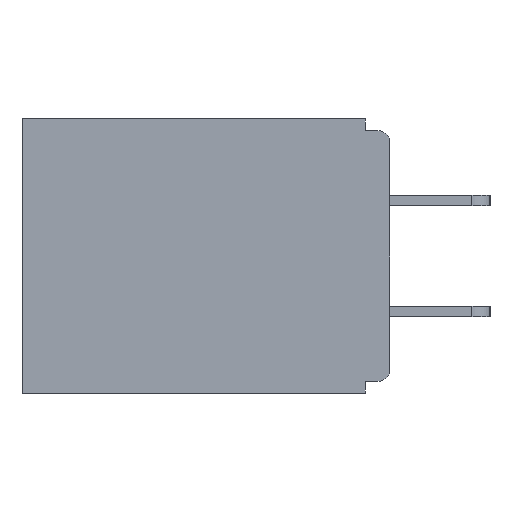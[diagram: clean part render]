
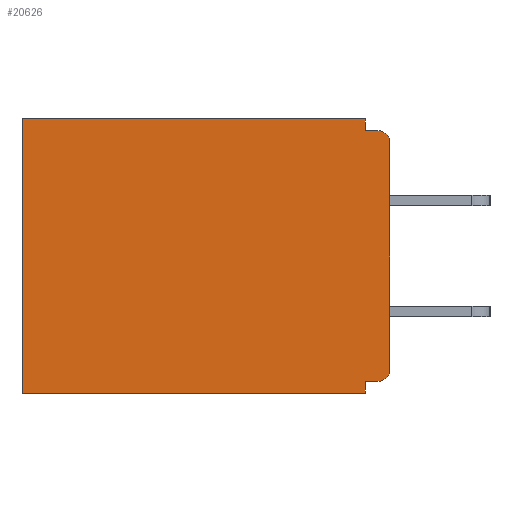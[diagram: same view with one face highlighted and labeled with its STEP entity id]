
A CAD part, left-side view. The second image highlights one B-rep face of the part: STEP entity #20626.
In plain terms, the highlighted planar face has unit normal (-1, 0, 0).
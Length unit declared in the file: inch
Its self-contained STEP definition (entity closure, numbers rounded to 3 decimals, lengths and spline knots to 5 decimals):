
#34 = DIRECTION ( 'NONE',  ( 0., -1., 0. ) ) ;
#69 = VERTEX_POINT ( 'NONE', #23006 ) ;
#91 = ORIENTED_EDGE ( 'NONE', *, *, #14475, .T. ) ;
#332 = DIRECTION ( 'NONE',  ( -1., 0., 0. ) ) ;
#580 = EDGE_CURVE ( 'NONE', #4819, #24319, #10371, .T. ) ;
#1262 = EDGE_CURVE ( 'NONE', #17373, #24319, #17213, .T. ) ;
#1753 = EDGE_CURVE ( 'NONE', #13020, #69, #8479, .T. ) ;
#2613 = EDGE_LOOP ( 'NONE', ( #17578, #21328, #8384, #18000, #91, #23982, #5837, #10115, #5992, #23986 ) ) ;
#3084 = EDGE_CURVE ( 'NONE', #17373, #24195, #9626, .T. ) ;
#3261 = VERTEX_POINT ( 'NONE', #17002 ) ;
#3632 = CARTESIAN_POINT ( 'NONE',  ( 0.298, 0., -0.313 ) ) ;
#3646 = FACE_OUTER_BOUND ( 'NONE', #2613, .T. ) ;
#4819 = VERTEX_POINT ( 'NONE', #14763 ) ;
#4847 = VECTOR ( 'NONE', #21313, 39.37008 ) ;
#5118 = VECTOR ( 'NONE', #14316, 39.37008 ) ;
#5837 = ORIENTED_EDGE ( 'NONE', *, *, #12443, .F. ) ;
#5872 = CARTESIAN_POINT ( 'NONE',  ( 0.298, 0.015, -0.03 ) ) ;
#5992 = ORIENTED_EDGE ( 'NONE', *, *, #580, .T. ) ;
#6903 = CARTESIAN_POINT ( 'NONE',  ( 0.298, 0.015, -0.313 ) ) ;
#7200 = CARTESIAN_POINT ( 'NONE',  ( 0.298, 0.015, -0.015 ) ) ;
#7772 = PLANE ( 'NONE',  #9525 ) ;
#8057 = VECTOR ( 'NONE', #10342, 39.37008 ) ;
#8081 = DIRECTION ( 'NONE',  ( 0., 0., -1. ) ) ;
#8384 = ORIENTED_EDGE ( 'NONE', *, *, #1753, .F. ) ;
#8479 = LINE ( 'NONE', #22284, #8778 ) ;
#8696 = EDGE_CURVE ( 'NONE', #69, #24195, #17627, .T. ) ;
#8778 = VECTOR ( 'NONE', #24211, 39.37008 ) ;
#8816 = DIRECTION ( 'NONE',  ( 0., 0., -1. ) ) ;
#8976 = DIRECTION ( 'NONE',  ( 0., 1., 0. ) ) ;
#9525 = AXIS2_PLACEMENT_3D ( 'NONE', #11665, #15156, #19032 ) ;
#9626 = CIRCLE ( 'NONE', #22221, 0.015 ) ;
#9645 = CARTESIAN_POINT ( 'NONE',  ( 0.298, 0., -0.015 ) ) ;
#10043 = EDGE_CURVE ( 'NONE', #13020, #17124, #18765, .T. ) ;
#10115 = ORIENTED_EDGE ( 'NONE', *, *, #12013, .F. ) ;
#10342 = DIRECTION ( 'NONE',  ( 0., 1., 0. ) ) ;
#10371 = CIRCLE ( 'NONE', #16552, 0.015 ) ;
#11306 = DIRECTION ( 'NONE',  ( 0., 1., 0. ) ) ;
#11663 = VECTOR ( 'NONE', #34, 39.37008 ) ;
#11665 = CARTESIAN_POINT ( 'NONE',  ( 0.298, 0., 0. ) ) ;
#11708 = CARTESIAN_POINT ( 'NONE',  ( 0.298, 0.46, 0. ) ) ;
#12013 = EDGE_CURVE ( 'NONE', #4819, #18906, #16290, .T. ) ;
#12443 = EDGE_CURVE ( 'NONE', #18906, #14614, #21073, .T. ) ;
#13020 = VERTEX_POINT ( 'NONE', #16680 ) ;
#13077 = DIRECTION ( 'NONE',  ( 0., 0., -1. ) ) ;
#13244 = CARTESIAN_POINT ( 'NONE',  ( 0.298, 0., 0. ) ) ;
#13925 = VECTOR ( 'NONE', #13077, 39.37008 ) ;
#13950 = CARTESIAN_POINT ( 'NONE',  ( 0.298, 0.46, 0. ) ) ;
#14316 = DIRECTION ( 'NONE',  ( 0., 0., -1. ) ) ;
#14475 = EDGE_CURVE ( 'NONE', #17124, #3261, #18993, .T. ) ;
#14614 = VERTEX_POINT ( 'NONE', #19566 ) ;
#14759 = CARTESIAN_POINT ( 'NONE',  ( 0.298, 0., -0.03 ) ) ;
#14763 = CARTESIAN_POINT ( 'NONE',  ( 0.298, 0.015, -0.328 ) ) ;
#14770 = CARTESIAN_POINT ( 'NONE',  ( 0.298, 0., -0.328 ) ) ;
#15156 = DIRECTION ( 'NONE',  ( 1., 0., 0. ) ) ;
#15453 = VECTOR ( 'NONE', #11306, 39.37008 ) ;
#16206 = CARTESIAN_POINT ( 'NONE',  ( 0.298, 0., -0.343 ) ) ;
#16290 = LINE ( 'NONE', #14770, #17485 ) ;
#16552 = AXIS2_PLACEMENT_3D ( 'NONE', #6903, #20321, #8816 ) ;
#16680 = CARTESIAN_POINT ( 'NONE',  ( 0.298, 0.031, 0. ) ) ;
#17002 = CARTESIAN_POINT ( 'NONE',  ( 0.298, 0.46, -0.343 ) ) ;
#17124 = VERTEX_POINT ( 'NONE', #13950 ) ;
#17213 = LINE ( 'NONE', #13244, #13925 ) ;
#17373 = VERTEX_POINT ( 'NONE', #14759 ) ;
#17485 = VECTOR ( 'NONE', #8976, 39.37008 ) ;
#17578 = ORIENTED_EDGE ( 'NONE', *, *, #3084, .T. ) ;
#17627 = LINE ( 'NONE', #9645, #11663 ) ;
#18000 = ORIENTED_EDGE ( 'NONE', *, *, #10043, .T. ) ;
#18765 = LINE ( 'NONE', #22789, #15453 ) ;
#18906 = VERTEX_POINT ( 'NONE', #24816 ) ;
#18993 = LINE ( 'NONE', #11708, #4847 ) ;
#19032 = DIRECTION ( 'NONE',  ( 0., 0., -1. ) ) ;
#19566 = CARTESIAN_POINT ( 'NONE',  ( 0.298, 0.031, -0.343 ) ) ;
#20321 = DIRECTION ( 'NONE',  ( -1., 0., 0. ) ) ;
#20353 = LINE ( 'NONE', #16206, #8057 ) ;
#20626 = ADVANCED_FACE ( 'NONE', ( #3646 ), #7772, .F. ) ;
#21073 = LINE ( 'NONE', #23812, #5118 ) ;
#21313 = DIRECTION ( 'NONE',  ( 0., 0., -1. ) ) ;
#21328 = ORIENTED_EDGE ( 'NONE', *, *, #8696, .F. ) ;
#22221 = AXIS2_PLACEMENT_3D ( 'NONE', #5872, #332, #8081 ) ;
#22284 = CARTESIAN_POINT ( 'NONE',  ( 0.298, 0.031, -0.343 ) ) ;
#22789 = CARTESIAN_POINT ( 'NONE',  ( 0.298, 0., 0. ) ) ;
#23006 = CARTESIAN_POINT ( 'NONE',  ( 0.298, 0.031, -0.015 ) ) ;
#23812 = CARTESIAN_POINT ( 'NONE',  ( 0.298, 0.031, -0.343 ) ) ;
#23955 = EDGE_CURVE ( 'NONE', #14614, #3261, #20353, .T. ) ;
#23982 = ORIENTED_EDGE ( 'NONE', *, *, #23955, .F. ) ;
#23986 = ORIENTED_EDGE ( 'NONE', *, *, #1262, .F. ) ;
#24195 = VERTEX_POINT ( 'NONE', #7200 ) ;
#24211 = DIRECTION ( 'NONE',  ( 0., 0., -1. ) ) ;
#24319 = VERTEX_POINT ( 'NONE', #3632 ) ;
#24816 = CARTESIAN_POINT ( 'NONE',  ( 0.298, 0.031, -0.328 ) ) ;
